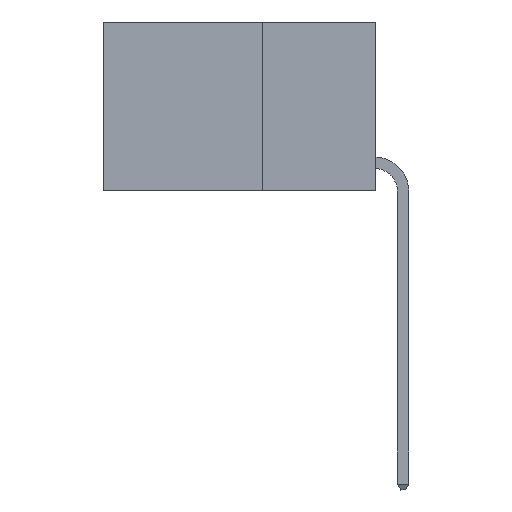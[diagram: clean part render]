
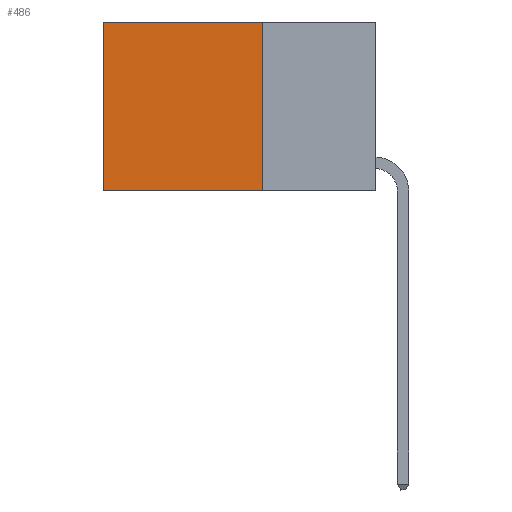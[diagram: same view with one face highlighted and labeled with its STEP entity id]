
A CAD part, left-side view. The second image highlights one B-rep face of the part: STEP entity #486.
In plain terms, the highlighted planar face has unit normal (-1, 0, 0).
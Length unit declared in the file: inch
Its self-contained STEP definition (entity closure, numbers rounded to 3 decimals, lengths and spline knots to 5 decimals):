
#403 = DIRECTION ( 'NONE',  ( 0., 0., -1. ) ) ;
#486 = ADVANCED_FACE ( 'NONE', ( #4619 ), #26708, .F. ) ;
#1040 = VERTEX_POINT ( 'NONE', #9638 ) ;
#2222 = VERTEX_POINT ( 'NONE', #9221 ) ;
#2777 = ORIENTED_EDGE ( 'NONE', *, *, #28234, .F. ) ;
#2981 = CARTESIAN_POINT ( 'NONE',  ( 0.2625, 0.6, 0. ) ) ;
#3054 = VECTOR ( 'NONE', #8262, 39.37008 ) ;
#3412 = VERTEX_POINT ( 'NONE', #20715 ) ;
#4619 = FACE_OUTER_BOUND ( 'NONE', #10252, .T. ) ;
#4907 = DIRECTION ( 'NONE',  ( 1., 0., 0. ) ) ;
#5004 = LINE ( 'NONE', #2981, #11631 ) ;
#6097 = LINE ( 'NONE', #12489, #28473 ) ;
#8262 = DIRECTION ( 'NONE',  ( 0., 1., 0. ) ) ;
#8826 = CARTESIAN_POINT ( 'NONE',  ( 0.2625, 0.25, -0.37 ) ) ;
#9221 = CARTESIAN_POINT ( 'NONE',  ( 0.2625, 0.6, 0. ) ) ;
#9252 = CARTESIAN_POINT ( 'NONE',  ( 0.2625, 0.25, 0. ) ) ;
#9638 = CARTESIAN_POINT ( 'NONE',  ( 0.2625, 0.6, -0.37 ) ) ;
#10252 = EDGE_LOOP ( 'NONE', ( #28297, #17181, #2777, #25677 ) ) ;
#11045 = AXIS2_PLACEMENT_3D ( 'NONE', #9252, #4907, #11565 ) ;
#11565 = DIRECTION ( 'NONE',  ( 0., 0., -1. ) ) ;
#11631 = VECTOR ( 'NONE', #403, 39.37008 ) ;
#11674 = VECTOR ( 'NONE', #17361, 39.37008 ) ;
#12489 = CARTESIAN_POINT ( 'NONE',  ( 0.2625, 0.25, 0. ) ) ;
#16578 = CARTESIAN_POINT ( 'NONE',  ( 0.2625, 0.25, 0. ) ) ;
#17181 = ORIENTED_EDGE ( 'NONE', *, *, #26870, .F. ) ;
#17361 = DIRECTION ( 'NONE',  ( 0., 1., 0. ) ) ;
#18151 = VERTEX_POINT ( 'NONE', #16578 ) ;
#18445 = EDGE_CURVE ( 'NONE', #2222, #1040, #5004, .T. ) ;
#19803 = LINE ( 'NONE', #28320, #11674 ) ;
#19963 = EDGE_CURVE ( 'NONE', #18151, #2222, #19803, .T. ) ;
#20715 = CARTESIAN_POINT ( 'NONE',  ( 0.2625, 0.25, -0.37 ) ) ;
#23436 = DIRECTION ( 'NONE',  ( 0., 0., -1. ) ) ;
#23714 = LINE ( 'NONE', #8826, #3054 ) ;
#25677 = ORIENTED_EDGE ( 'NONE', *, *, #19963, .T. ) ;
#26708 = PLANE ( 'NONE',  #11045 ) ;
#26870 = EDGE_CURVE ( 'NONE', #3412, #1040, #23714, .T. ) ;
#28234 = EDGE_CURVE ( 'NONE', #18151, #3412, #6097, .T. ) ;
#28297 = ORIENTED_EDGE ( 'NONE', *, *, #18445, .T. ) ;
#28320 = CARTESIAN_POINT ( 'NONE',  ( 0.2625, 0.25, 0. ) ) ;
#28473 = VECTOR ( 'NONE', #23436, 39.37008 ) ;
